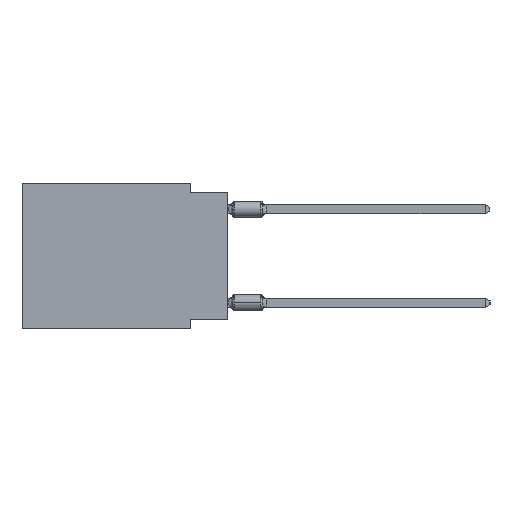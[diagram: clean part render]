
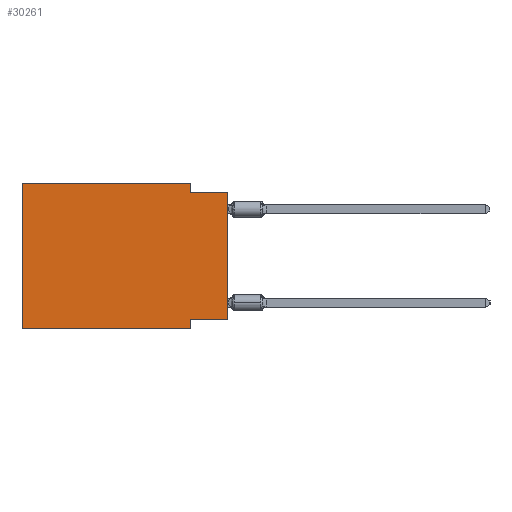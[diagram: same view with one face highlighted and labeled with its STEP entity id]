
A CAD part, left-side view. The second image highlights one B-rep face of the part: STEP entity #30261.
In plain terms, the highlighted planar face has unit normal (-1, 0, 0).
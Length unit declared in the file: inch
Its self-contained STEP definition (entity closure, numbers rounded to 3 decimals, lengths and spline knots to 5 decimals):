
#295 = VERTEX_POINT ( 'NONE', #2302 ) ;
#428 = VECTOR ( 'NONE', #18333, 39.37008 ) ;
#436 = DIRECTION ( 'NONE',  ( 0., 0., -1. ) ) ;
#513 = CARTESIAN_POINT ( 'NONE',  ( 0., 0.1, -0.39 ) ) ;
#808 = LINE ( 'NONE', #10402, #24089 ) ;
#2302 = CARTESIAN_POINT ( 'NONE',  ( 0., 0.55, -0.39 ) ) ;
#2417 = EDGE_LOOP ( 'NONE', ( #26497, #7723, #20899, #19126, #25469, #5240, #14169, #15321 ) ) ;
#3667 = CARTESIAN_POINT ( 'NONE',  ( 0., 0.55, -0.39 ) ) ;
#4447 = VERTEX_POINT ( 'NONE', #26445 ) ;
#5047 = CARTESIAN_POINT ( 'NONE',  ( 0., 0., -0.365 ) ) ;
#5095 = LINE ( 'NONE', #513, #18373 ) ;
#5103 = EDGE_CURVE ( 'NONE', #13563, #5914, #20722, .T. ) ;
#5240 = ORIENTED_EDGE ( 'NONE', *, *, #29423, .T. ) ;
#5393 = CARTESIAN_POINT ( 'NONE',  ( 0., 0., 0. ) ) ;
#5914 = VERTEX_POINT ( 'NONE', #9218 ) ;
#6988 = DIRECTION ( 'NONE',  ( 0., 0., -1. ) ) ;
#7723 = ORIENTED_EDGE ( 'NONE', *, *, #27028, .F. ) ;
#8032 = VECTOR ( 'NONE', #22681, 39.37008 ) ;
#8666 = VECTOR ( 'NONE', #25909, 39.37008 ) ;
#9218 = CARTESIAN_POINT ( 'NONE',  ( 0., 0.1, -0.365 ) ) ;
#10033 = CARTESIAN_POINT ( 'NONE',  ( 0., 0.55, 0. ) ) ;
#10402 = CARTESIAN_POINT ( 'NONE',  ( 0., 0.1, 0. ) ) ;
#12417 = DIRECTION ( 'NONE',  ( 1., 0., 0. ) ) ;
#12602 = EDGE_CURVE ( 'NONE', #4447, #31168, #18073, .T. ) ;
#13190 = EDGE_CURVE ( 'NONE', #5914, #16205, #5095, .T. ) ;
#13563 = VERTEX_POINT ( 'NONE', #5047 ) ;
#13795 = CARTESIAN_POINT ( 'NONE',  ( 0., 0.55, 0. ) ) ;
#14042 = CARTESIAN_POINT ( 'NONE',  ( 0., 0., -0.025 ) ) ;
#14169 = ORIENTED_EDGE ( 'NONE', *, *, #13190, .F. ) ;
#14266 = EDGE_CURVE ( 'NONE', #31168, #26163, #808, .T. ) ;
#14271 = DIRECTION ( 'NONE',  ( 0., 0., -1. ) ) ;
#15321 = ORIENTED_EDGE ( 'NONE', *, *, #5103, .F. ) ;
#15847 = VECTOR ( 'NONE', #26353, 39.37008 ) ;
#16205 = VERTEX_POINT ( 'NONE', #30924 ) ;
#16552 = LINE ( 'NONE', #14042, #15847 ) ;
#18012 = CARTESIAN_POINT ( 'NONE',  ( 0., 0.1, -0.025 ) ) ;
#18073 = LINE ( 'NONE', #20448, #8032 ) ;
#18333 = DIRECTION ( 'NONE',  ( 0., -1., 0. ) ) ;
#18341 = CARTESIAN_POINT ( 'NONE',  ( 0., 0., -0.365 ) ) ;
#18373 = VECTOR ( 'NONE', #6988, 39.37008 ) ;
#19126 = ORIENTED_EDGE ( 'NONE', *, *, #12602, .F. ) ;
#19592 = DIRECTION ( 'NONE',  ( 0., 0., 1. ) ) ;
#19749 = LINE ( 'NONE', #5393, #23439 ) ;
#20448 = CARTESIAN_POINT ( 'NONE',  ( 0., 0.55, 0. ) ) ;
#20722 = LINE ( 'NONE', #18341, #8666 ) ;
#20899 = ORIENTED_EDGE ( 'NONE', *, *, #14266, .F. ) ;
#21419 = EDGE_CURVE ( 'NONE', #295, #4447, #25769, .T. ) ;
#22669 = AXIS2_PLACEMENT_3D ( 'NONE', #10033, #12417, #436 ) ;
#22681 = DIRECTION ( 'NONE',  ( 0., -1., 0. ) ) ;
#22722 = CARTESIAN_POINT ( 'NONE',  ( 0., 0.1, 0. ) ) ;
#23428 = DIRECTION ( 'NONE',  ( 0., 0., 1. ) ) ;
#23439 = VECTOR ( 'NONE', #19592, 39.37008 ) ;
#24089 = VECTOR ( 'NONE', #14271, 39.37008 ) ;
#24721 = PLANE ( 'NONE',  #22669 ) ;
#25275 = LINE ( 'NONE', #3667, #428 ) ;
#25469 = ORIENTED_EDGE ( 'NONE', *, *, #21419, .F. ) ;
#25769 = LINE ( 'NONE', #13795, #29294 ) ;
#25909 = DIRECTION ( 'NONE',  ( 0., 1., 0. ) ) ;
#26163 = VERTEX_POINT ( 'NONE', #18012 ) ;
#26353 = DIRECTION ( 'NONE',  ( 0., -1., 0. ) ) ;
#26445 = CARTESIAN_POINT ( 'NONE',  ( 0., 0.55, 0. ) ) ;
#26497 = ORIENTED_EDGE ( 'NONE', *, *, #26833, .T. ) ;
#26833 = EDGE_CURVE ( 'NONE', #13563, #26853, #19749, .T. ) ;
#26853 = VERTEX_POINT ( 'NONE', #29387 ) ;
#27028 = EDGE_CURVE ( 'NONE', #26163, #26853, #16552, .T. ) ;
#28009 = FACE_OUTER_BOUND ( 'NONE', #2417, .T. ) ;
#29294 = VECTOR ( 'NONE', #23428, 39.37008 ) ;
#29387 = CARTESIAN_POINT ( 'NONE',  ( 0., 0., -0.025 ) ) ;
#29423 = EDGE_CURVE ( 'NONE', #295, #16205, #25275, .T. ) ;
#30261 = ADVANCED_FACE ( 'NONE', ( #28009 ), #24721, .F. ) ;
#30924 = CARTESIAN_POINT ( 'NONE',  ( 0., 0.1, -0.39 ) ) ;
#31168 = VERTEX_POINT ( 'NONE', #22722 ) ;
